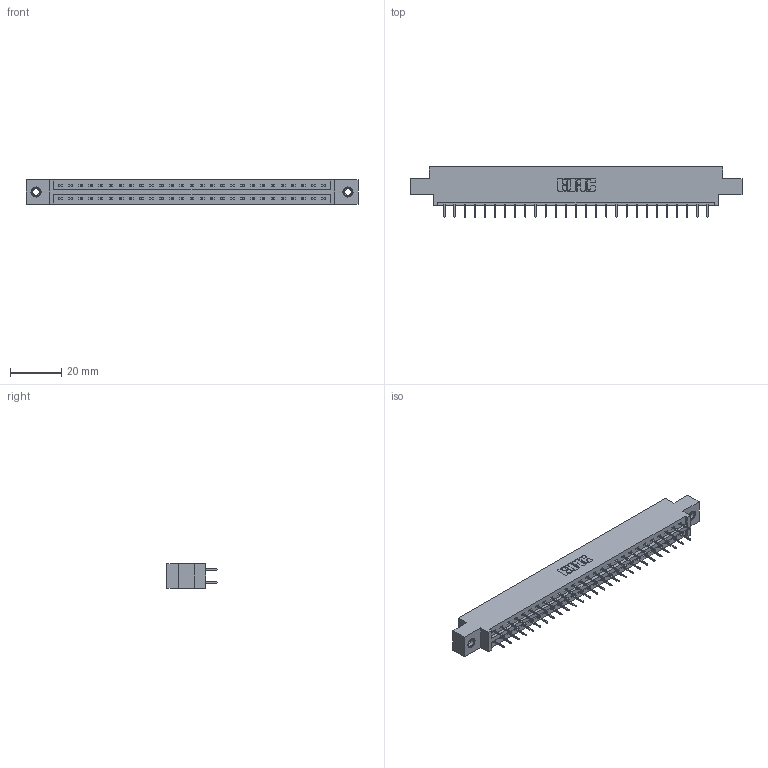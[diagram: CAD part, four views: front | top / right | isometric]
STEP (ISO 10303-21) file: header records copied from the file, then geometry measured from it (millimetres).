
FILE_DESCRIPTION (( 'STEP AP203' ), '1' );
FILE_NAME ('387-054-524-807.STEP', '2019-10-19T04:47:20', ( '' ), ( '' ), 'SwSTEP 2.0', 'SolidWorks 2016', '' );
FILE_SCHEMA (( 'CONFIG_CONTROL_DESIGN' ));
Length unit declared in the file: inch
Products named in the file (4): 337 Part_0.170 Offset - 0.156 Dia-TI; 387-054-524-807; 345-250-001_345-250-005-103; 345-292-001_345-293-124
Assembly tree (57 placements, depth 2):
  387-054-524-807
    337 Part_0.170 Offset - 0.156 Dia-TI
    345-292-001_345-293-124  x54
    345-250-001_345-250-005-103  x2
Bounding box: 130 x 19.69 x 9.4 mm (x, y, z)
Volume: 13287.7 mm3; surface area: 14766.8 mm2
Topology: 57 solids, 57 shells, 3310 faces, 9369 edges, 6022 vertices
Faces by surface type: plane 2482, cylinder 812, cone 12, torus 4
Entity records: 24266 total; most frequent: CARTESIAN_POINT 4081, ORIENTED_EDGE 4010, DIRECTION 3531, EDGE_CURVE 2005, VECTOR 1861, LINE 1861, VERTEX_POINT 1328, AXIS2_PLACEMENT_3D 835
